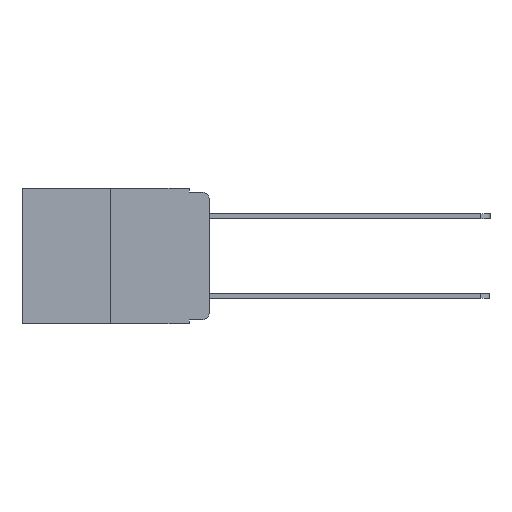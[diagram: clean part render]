
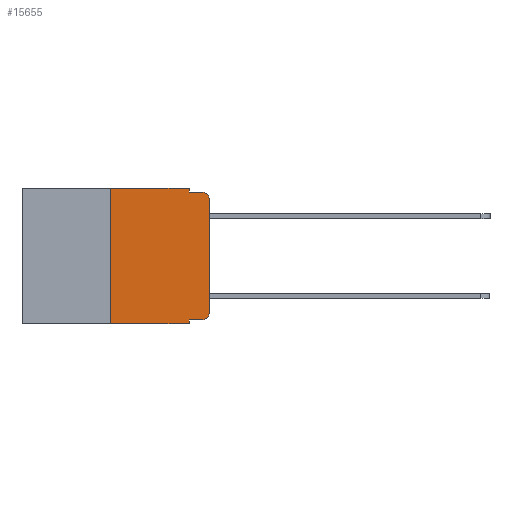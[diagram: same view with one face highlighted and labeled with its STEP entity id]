
A CAD part, left-side view. The second image highlights one B-rep face of the part: STEP entity #15655.
In plain terms, the highlighted planar face has unit normal (-1, 0, 0).
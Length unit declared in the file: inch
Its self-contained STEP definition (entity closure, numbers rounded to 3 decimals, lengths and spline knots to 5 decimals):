
#235 = VERTEX_POINT ( 'NONE', #5262 ) ;
#361 = CARTESIAN_POINT ( 'NONE',  ( 0., 0.25, 0. ) ) ;
#899 = VERTEX_POINT ( 'NONE', #361 ) ;
#951 = DIRECTION ( 'NONE',  ( 0., -1., 0. ) ) ;
#1179 = EDGE_LOOP ( 'NONE', ( #11164, #7216, #18193, #14299, #11961, #21314, #14576, #6205, #4414, #4926 ) ) ;
#1222 = FACE_OUTER_BOUND ( 'NONE', #1179, .T. ) ;
#1254 = LINE ( 'NONE', #15354, #18477 ) ;
#1768 = VERTEX_POINT ( 'NONE', #19033 ) ;
#2396 = CARTESIAN_POINT ( 'NONE',  ( 0., 0., -0.313 ) ) ;
#2732 = EDGE_CURVE ( 'NONE', #17581, #7437, #10157, .T. ) ;
#2800 = CARTESIAN_POINT ( 'NONE',  ( 0., 0.051, -0.333 ) ) ;
#3100 = VERTEX_POINT ( 'NONE', #5235 ) ;
#3125 = LINE ( 'NONE', #3888, #15908 ) ;
#3271 = EDGE_CURVE ( 'NONE', #14084, #1768, #3428, .T. ) ;
#3389 = CARTESIAN_POINT ( 'NONE',  ( 0., 0.02, -0.333 ) ) ;
#3428 = CIRCLE ( 'NONE', #13239, 0.02 ) ;
#3888 = CARTESIAN_POINT ( 'NONE',  ( 0., 0.473, -0.343 ) ) ;
#4167 = DIRECTION ( 'NONE',  ( -1., 0., 0. ) ) ;
#4233 = LINE ( 'NONE', #21193, #21410 ) ;
#4414 = ORIENTED_EDGE ( 'NONE', *, *, #2732, .T. ) ;
#4732 = DIRECTION ( 'NONE',  ( 0., 0., -1. ) ) ;
#4926 = ORIENTED_EDGE ( 'NONE', *, *, #10198, .T. ) ;
#5029 = VERTEX_POINT ( 'NONE', #15074 ) ;
#5128 = AXIS2_PLACEMENT_3D ( 'NONE', #12003, #8700, #20349 ) ;
#5235 = CARTESIAN_POINT ( 'NONE',  ( 0., 0.051, -0.343 ) ) ;
#5262 = CARTESIAN_POINT ( 'NONE',  ( 0., 0.051, -0.01 ) ) ;
#5375 = EDGE_CURVE ( 'NONE', #17581, #3100, #9299, .T. ) ;
#5727 = VERTEX_POINT ( 'NONE', #12077 ) ;
#5908 = CARTESIAN_POINT ( 'NONE',  ( 0., 0.473, 0. ) ) ;
#6205 = ORIENTED_EDGE ( 'NONE', *, *, #5375, .F. ) ;
#6284 = CARTESIAN_POINT ( 'NONE',  ( 0., 0., -0.03 ) ) ;
#6668 = VECTOR ( 'NONE', #19524, 39.37008 ) ;
#7216 = ORIENTED_EDGE ( 'NONE', *, *, #3271, .T. ) ;
#7437 = VERTEX_POINT ( 'NONE', #3389 ) ;
#7807 = EDGE_CURVE ( 'NONE', #899, #5727, #17020, .T. ) ;
#8005 = AXIS2_PLACEMENT_3D ( 'NONE', #14143, #4167, #15835 ) ;
#8700 = DIRECTION ( 'NONE',  ( 1., 0., 0. ) ) ;
#9267 = DIRECTION ( 'NONE',  ( 0., 0., -1. ) ) ;
#9299 = LINE ( 'NONE', #20945, #17160 ) ;
#9432 = EDGE_CURVE ( 'NONE', #13312, #14084, #1254, .T. ) ;
#10157 = LINE ( 'NONE', #18002, #13583 ) ;
#10198 = EDGE_CURVE ( 'NONE', #7437, #13312, #18167, .T. ) ;
#10360 = EDGE_CURVE ( 'NONE', #5727, #235, #19973, .T. ) ;
#10502 = DIRECTION ( 'NONE',  ( 0., -1., 0. ) ) ;
#11164 = ORIENTED_EDGE ( 'NONE', *, *, #9432, .T. ) ;
#11239 = DIRECTION ( 'NONE',  ( 0., -1., 0. ) ) ;
#11304 = CARTESIAN_POINT ( 'NONE',  ( 0., 0.25, 0. ) ) ;
#11677 = VECTOR ( 'NONE', #12968, 39.37008 ) ;
#11961 = ORIENTED_EDGE ( 'NONE', *, *, #7807, .F. ) ;
#12003 = CARTESIAN_POINT ( 'NONE',  ( 0., 0.473, 0. ) ) ;
#12077 = CARTESIAN_POINT ( 'NONE',  ( 0., 0.051, 0. ) ) ;
#12181 = DIRECTION ( 'NONE',  ( 0., -1., 0. ) ) ;
#12968 = DIRECTION ( 'NONE',  ( 0., 0., 1. ) ) ;
#13016 = EDGE_CURVE ( 'NONE', #235, #1768, #4233, .T. ) ;
#13239 = AXIS2_PLACEMENT_3D ( 'NONE', #17417, #17124, #4732 ) ;
#13312 = VERTEX_POINT ( 'NONE', #2396 ) ;
#13583 = VECTOR ( 'NONE', #12181, 39.37008 ) ;
#14084 = VERTEX_POINT ( 'NONE', #6284 ) ;
#14143 = CARTESIAN_POINT ( 'NONE',  ( 0., 0.02, -0.313 ) ) ;
#14299 = ORIENTED_EDGE ( 'NONE', *, *, #10360, .F. ) ;
#14455 = EDGE_CURVE ( 'NONE', #5029, #3100, #3125, .T. ) ;
#14576 = ORIENTED_EDGE ( 'NONE', *, *, #14455, .T. ) ;
#15074 = CARTESIAN_POINT ( 'NONE',  ( 0., 0.25, -0.343 ) ) ;
#15354 = CARTESIAN_POINT ( 'NONE',  ( 0., 0., 0. ) ) ;
#15655 = ADVANCED_FACE ( 'NONE', ( #1222 ), #17042, .F. ) ;
#15835 = DIRECTION ( 'NONE',  ( 0., 0., -1. ) ) ;
#15908 = VECTOR ( 'NONE', #10502, 39.37008 ) ;
#17020 = LINE ( 'NONE', #5908, #21404 ) ;
#17040 = DIRECTION ( 'NONE',  ( 0., 0., 1. ) ) ;
#17042 = PLANE ( 'NONE',  #5128 ) ;
#17124 = DIRECTION ( 'NONE',  ( -1., 0., 0. ) ) ;
#17160 = VECTOR ( 'NONE', #9267, 39.37008 ) ;
#17417 = CARTESIAN_POINT ( 'NONE',  ( 0., 0.02, -0.03 ) ) ;
#17581 = VERTEX_POINT ( 'NONE', #2800 ) ;
#17673 = LINE ( 'NONE', #11304, #11677 ) ;
#17860 = CARTESIAN_POINT ( 'NONE',  ( 0., 0.051, 0. ) ) ;
#18002 = CARTESIAN_POINT ( 'NONE',  ( 0., 0.051, -0.333 ) ) ;
#18167 = CIRCLE ( 'NONE', #8005, 0.02 ) ;
#18193 = ORIENTED_EDGE ( 'NONE', *, *, #13016, .F. ) ;
#18477 = VECTOR ( 'NONE', #17040, 39.37008 ) ;
#19033 = CARTESIAN_POINT ( 'NONE',  ( 0., 0.02, -0.01 ) ) ;
#19524 = DIRECTION ( 'NONE',  ( 0., 0., -1. ) ) ;
#19973 = LINE ( 'NONE', #17860, #6668 ) ;
#20349 = DIRECTION ( 'NONE',  ( 0., 0., -1. ) ) ;
#20706 = EDGE_CURVE ( 'NONE', #5029, #899, #17673, .T. ) ;
#20945 = CARTESIAN_POINT ( 'NONE',  ( 0., 0.051, 0. ) ) ;
#21193 = CARTESIAN_POINT ( 'NONE',  ( 0., 0.051, -0.01 ) ) ;
#21314 = ORIENTED_EDGE ( 'NONE', *, *, #20706, .F. ) ;
#21404 = VECTOR ( 'NONE', #951, 39.37008 ) ;
#21410 = VECTOR ( 'NONE', #11239, 39.37008 ) ;
